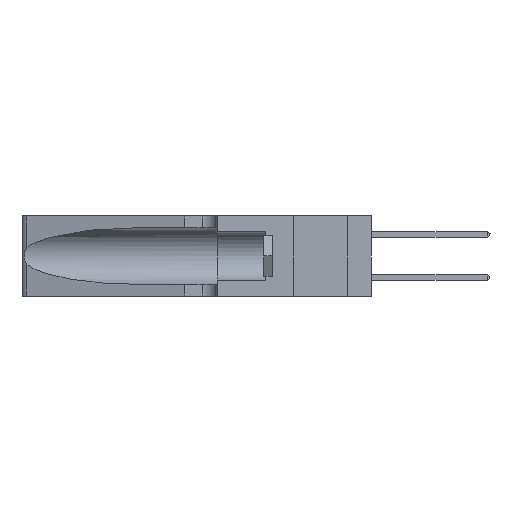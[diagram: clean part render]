
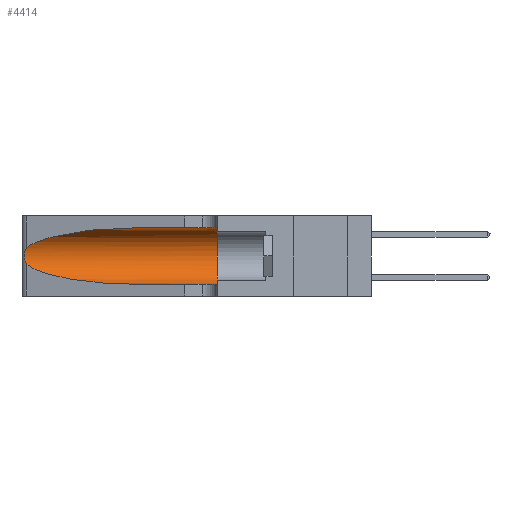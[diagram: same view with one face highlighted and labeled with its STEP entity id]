
A CAD part, left-side view. The second image highlights one B-rep face of the part: STEP entity #4414.
In plain terms, the highlighted cylindrical face has radius 3.308 mm (diameter 6.617 mm), a partial arc.
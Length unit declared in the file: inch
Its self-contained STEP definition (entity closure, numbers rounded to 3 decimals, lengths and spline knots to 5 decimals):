
#1353 = EDGE_CURVE ( 'NONE', #26856, #24091, #24297, .T. ) ;
#1788 = EDGE_CURVE ( 'NONE', #26856, #13291, #11720, .T. ) ;
#2182 = DIRECTION ( 'NONE',  ( 0., 0., 1. ) ) ;
#2241 = ORIENTED_EDGE ( 'NONE', *, *, #11519, .T. ) ;
#2689 = CARTESIAN_POINT ( 'NONE',  ( 0.2373, 1.15595, 0.28018 ) ) ;
#2922 = DIRECTION ( 'NONE',  ( 0., 0., -1. ) ) ;
#2943 = CARTESIAN_POINT ( 'NONE',  ( 0.26017, 1.23833, 0.17102 ) ) ;
#4159 = DIRECTION ( 'NONE',  ( 0., -1., 0. ) ) ;
#4414 = ADVANCED_FACE ( 'NONE', ( #37914 ), #35891, .F. ) ;
#4947 = CARTESIAN_POINT ( 'NONE',  ( 0.1305, 0.72297, 0.05475 ) ) ;
#6218 = CARTESIAN_POINT ( 'NONE',  ( 0.25789, 1.23486, 0.15765 ) ) ;
#8450 = CIRCLE ( 'NONE', #33180, 0.13025 ) ;
#8694 = CARTESIAN_POINT ( 'NONE',  ( 0.1305, 0.35, 0.31525 ) ) ;
#8830 = CARTESIAN_POINT ( 'NONE',  ( 0.1305, 0.72297, 0.05475 ) ) ;
#9202 = ORIENTED_EDGE ( 'NONE', *, *, #12324, .T. ) ;
#9555 = CARTESIAN_POINT ( 'NONE',  ( 0.25555, 1.22993, 0.14849 ) ) ;
#11391 = EDGE_CURVE ( 'NONE', #37039, #36149, #31446, .T. ) ;
#11519 = EDGE_CURVE ( 'NONE', #13291, #37039, #23822, .T. ) ;
#11720 =( BOUNDED_CURVE ( )  B_SPLINE_CURVE ( 3, ( #22341, #25635, #2689, #28934 ),
 .UNSPECIFIED., .F., .F. ) 
 B_SPLINE_CURVE_WITH_KNOTS ( ( 4, 4 ),
 ( 1.5708, 2.84003 ),
 .UNSPECIFIED. ) 
 CURVE ( )  GEOMETRIC_REPRESENTATION_ITEM ( )  RATIONAL_B_SPLINE_CURVE ( ( 1., 0.87, 0.87, 1. ) ) 
 REPRESENTATION_ITEM ( '' )  );
#12324 = EDGE_CURVE ( 'NONE', #36149, #19162, #18459, .T. ) ;
#13088 = EDGE_LOOP ( 'NONE', ( #32499, #2241, #20790, #9202, #21120, #32888 ) ) ;
#13291 = VERTEX_POINT ( 'NONE', #27047 ) ;
#15570 = VECTOR ( 'NONE', #36660, 39.37008 ) ;
#15846 = CARTESIAN_POINT ( 'NONE',  ( 0.25555, 1.22994, 0.2215 ) ) ;
#15989 = CARTESIAN_POINT ( 'NONE',  ( 0.25787, 1.23484, 0.2124 ) ) ;
#17443 = VECTOR ( 'NONE', #4159, 39.37008 ) ;
#18459 = LINE ( 'NONE', #33687, #17443 ) ;
#19162 = VERTEX_POINT ( 'NONE', #31874 ) ;
#19294 = CARTESIAN_POINT ( 'NONE',  ( 0.26018, 1.23835, 0.19895 ) ) ;
#20790 = ORIENTED_EDGE ( 'NONE', *, *, #11391, .T. ) ;
#21120 = ORIENTED_EDGE ( 'NONE', *, *, #24773, .F. ) ;
#21828 = DIRECTION ( 'NONE',  ( 0., 1., 0. ) ) ;
#21882 = CARTESIAN_POINT ( 'NONE',  ( 0.18966, 0.96281, 0.05475 ) ) ;
#22341 = CARTESIAN_POINT ( 'NONE',  ( 0.1305, 0.72297, 0.31525 ) ) ;
#22574 = DIRECTION ( 'NONE',  ( 0., -1., 0. ) ) ;
#22603 = CARTESIAN_POINT ( 'NONE',  ( 0.26075, 1.23896, 0.178 ) ) ;
#23497 = CARTESIAN_POINT ( 'NONE',  ( 0.1305, 1.61858, 0.31525 ) ) ;
#23822 = B_SPLINE_CURVE_WITH_KNOTS ( 'NONE', 3,
 ( #32347, #15846, #35615, #15989, #38882, #19294, #42176, #22603, #2943, #25874, #6218, #29190, #9555, #32484 ),
 .UNSPECIFIED., .F., .F.,
 ( 4, 2, 2, 2, 2, 2, 4 ),
 ( 0., 0.00027, 0.00053, 0.00107, 0.0016, 0.00187, 0.00214 ),
 .UNSPECIFIED. ) ;
#24091 = VERTEX_POINT ( 'NONE', #8694 ) ;
#24297 = LINE ( 'NONE', #23497, #15570 ) ;
#24773 = EDGE_CURVE ( 'NONE', #24091, #19162, #8450, .T. ) ;
#25635 = CARTESIAN_POINT ( 'NONE',  ( 0.18966, 0.96281, 0.31525 ) ) ;
#25860 = CARTESIAN_POINT ( 'NONE',  ( 0.1305, 1.61858, 0.185 ) ) ;
#25874 = CARTESIAN_POINT ( 'NONE',  ( 0.25856, 1.23593, 0.16098 ) ) ;
#26774 = CARTESIAN_POINT ( 'NONE',  ( 0.1305, 0.72297, 0.31525 ) ) ;
#26856 = VERTEX_POINT ( 'NONE', #26774 ) ;
#27047 = CARTESIAN_POINT ( 'NONE',  ( 0.25487, 1.22718, 0.22369 ) ) ;
#28470 = CARTESIAN_POINT ( 'NONE',  ( 0.25487, 1.22718, 0.14631 ) ) ;
#28843 = CARTESIAN_POINT ( 'NONE',  ( 0.25487, 1.22718, 0.14631 ) ) ;
#28934 = CARTESIAN_POINT ( 'NONE',  ( 0.25487, 1.22718, 0.22369 ) ) ;
#29190 = CARTESIAN_POINT ( 'NONE',  ( 0.25639, 1.23186, 0.15144 ) ) ;
#31446 =( BOUNDED_CURVE ( )  B_SPLINE_CURVE ( 3, ( #28470, #41471, #21882, #8830 ),
 .UNSPECIFIED., .F., .F. ) 
 B_SPLINE_CURVE_WITH_KNOTS ( ( 4, 4 ),
 ( 3.44316, 4.71239 ),
 .UNSPECIFIED. ) 
 CURVE ( )  GEOMETRIC_REPRESENTATION_ITEM ( )  RATIONAL_B_SPLINE_CURVE ( ( 1., 0.87, 0.87, 1. ) ) 
 REPRESENTATION_ITEM ( '' )  );
#31874 = CARTESIAN_POINT ( 'NONE',  ( 0.1305, 0.35, 0.05475 ) ) ;
#32347 = CARTESIAN_POINT ( 'NONE',  ( 0.25487, 1.22718, 0.22369 ) ) ;
#32484 = CARTESIAN_POINT ( 'NONE',  ( 0.25487, 1.22718, 0.14631 ) ) ;
#32499 = ORIENTED_EDGE ( 'NONE', *, *, #1788, .T. ) ;
#32888 = ORIENTED_EDGE ( 'NONE', *, *, #1353, .F. ) ;
#33180 = AXIS2_PLACEMENT_3D ( 'NONE', #41432, #21828, #2182 ) ;
#33687 = CARTESIAN_POINT ( 'NONE',  ( 0.1305, 1.61858, 0.05475 ) ) ;
#35056 = AXIS2_PLACEMENT_3D ( 'NONE', #25860, #22574, #2922 ) ;
#35615 = CARTESIAN_POINT ( 'NONE',  ( 0.25639, 1.23184, 0.21858 ) ) ;
#35891 = CYLINDRICAL_SURFACE ( 'NONE', #35056, 0.13025 ) ;
#36149 = VERTEX_POINT ( 'NONE', #4947 ) ;
#36660 = DIRECTION ( 'NONE',  ( 0., -1., 0. ) ) ;
#37039 = VERTEX_POINT ( 'NONE', #28843 ) ;
#37914 = FACE_OUTER_BOUND ( 'NONE', #13088, .T. ) ;
#38882 = CARTESIAN_POINT ( 'NONE',  ( 0.25854, 1.2359, 0.20912 ) ) ;
#41432 = CARTESIAN_POINT ( 'NONE',  ( 0.1305, 0.35, 0.185 ) ) ;
#41471 = CARTESIAN_POINT ( 'NONE',  ( 0.2373, 1.15595, 0.08982 ) ) ;
#42176 = CARTESIAN_POINT ( 'NONE',  ( 0.26075, 1.23896, 0.19203 ) ) ;
